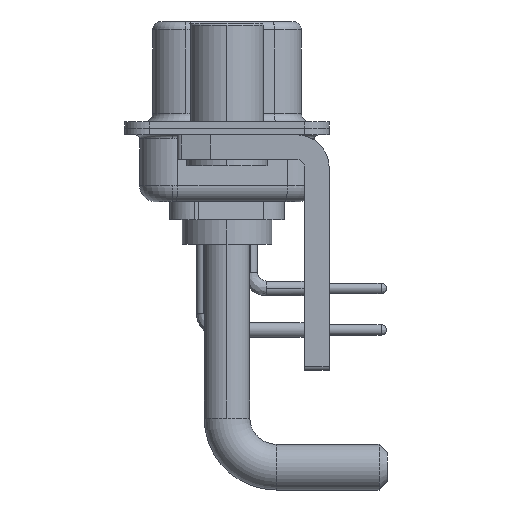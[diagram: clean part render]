
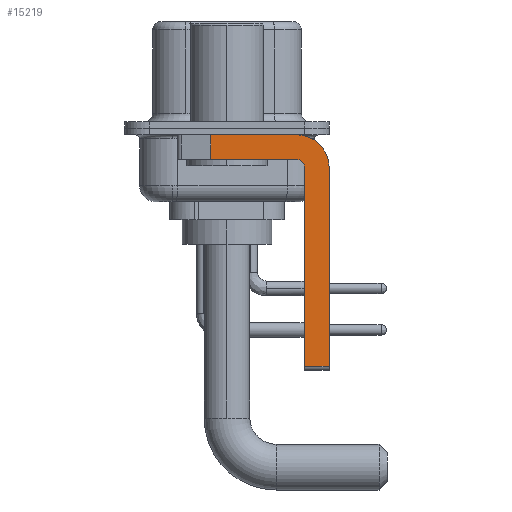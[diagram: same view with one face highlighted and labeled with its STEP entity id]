
A CAD part, left-side view. The second image highlights one B-rep face of the part: STEP entity #15219.
In plain terms, the highlighted planar face has unit normal (-1, 0, 0).
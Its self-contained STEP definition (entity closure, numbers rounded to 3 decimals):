
#39 = VERTEX_POINT ( 'NONE', #13458 ) ;
#466 = VERTEX_POINT ( 'NONE', #19669 ) ;
#591 = EDGE_CURVE ( 'NONE', #25137, #39, #25236, .T. ) ;
#1437 = DIRECTION ( 'NONE',  ( 0., 0., -1. ) ) ;
#1452 = EDGE_CURVE ( 'NONE', #3935, #466, #29299, .T. ) ;
#1576 = VERTEX_POINT ( 'NONE', #20144 ) ;
#1578 = PLANE ( 'NONE',  #26628 ) ;
#1872 = ORIENTED_EDGE ( 'NONE', *, *, #3422, .F. ) ;
#2029 = VERTEX_POINT ( 'NONE', #25623 ) ;
#2745 = VERTEX_POINT ( 'NONE', #3814 ) ;
#3008 = DIRECTION ( 'NONE',  ( 0., 0., -1. ) ) ;
#3422 = EDGE_CURVE ( 'NONE', #1576, #10425, #16753, .T. ) ;
#3678 = DIRECTION ( 'NONE',  ( 1., 0., 0. ) ) ;
#3814 = CARTESIAN_POINT ( 'NONE',  ( -2.9, -6.25, -14.55 ) ) ;
#3935 = VERTEX_POINT ( 'NONE', #21725 ) ;
#3974 = DIRECTION ( 'NONE',  ( 0., 1., 0. ) ) ;
#4480 = CIRCLE ( 'NONE', #8739, 2. ) ;
#4920 = ORIENTED_EDGE ( 'NONE', *, *, #23423, .F. ) ;
#5071 = AXIS2_PLACEMENT_3D ( 'NONE', #21309, #20336, #18812 ) ;
#6153 = EDGE_CURVE ( 'NONE', #10425, #2029, #4480, .T. ) ;
#6484 = CIRCLE ( 'NONE', #5071, 0.5 ) ;
#6546 = EDGE_CURVE ( 'NONE', #1576, #466, #14475, .T. ) ;
#6568 = ORIENTED_EDGE ( 'NONE', *, *, #1452, .F. ) ;
#7498 = ORIENTED_EDGE ( 'NONE', *, *, #591, .F. ) ;
#8739 = AXIS2_PLACEMENT_3D ( 'NONE', #9708, #23617, #3008 ) ;
#8880 = VECTOR ( 'NONE', #9494, 1000. ) ;
#8999 = VECTOR ( 'NONE', #3974, 1000. ) ;
#9494 = DIRECTION ( 'NONE',  ( 0., -1., 0. ) ) ;
#9590 = DIRECTION ( 'NONE',  ( 0., 0., -1. ) ) ;
#9708 = CARTESIAN_POINT ( 'NONE',  ( -2.9, -4.25, -2.4 ) ) ;
#10425 = VERTEX_POINT ( 'NONE', #23174 ) ;
#10518 = ORIENTED_EDGE ( 'NONE', *, *, #24227, .T. ) ;
#11633 = LINE ( 'NONE', #28333, #24427 ) ;
#11795 = CARTESIAN_POINT ( 'NONE',  ( -2.9, 0.978, -1.9 ) ) ;
#13458 = CARTESIAN_POINT ( 'NONE',  ( -2.9, -4.75, -2.4 ) ) ;
#14475 = LINE ( 'NONE', #11795, #28120 ) ;
#14942 = ORIENTED_EDGE ( 'NONE', *, *, #29248, .F. ) ;
#15219 = ADVANCED_FACE ( 'NONE', ( #26167 ), #1578, .F. ) ;
#16158 = CARTESIAN_POINT ( 'NONE',  ( -2.9, -4.25, -14.55 ) ) ;
#16207 = ORIENTED_EDGE ( 'NONE', *, *, #6153, .F. ) ;
#16385 = CARTESIAN_POINT ( 'NONE',  ( -2.9, -4.75, -14.8 ) ) ;
#16618 = CARTESIAN_POINT ( 'NONE',  ( -2.9, 3., -0.4 ) ) ;
#16753 = LINE ( 'NONE', #16618, #24678 ) ;
#17093 = DIRECTION ( 'NONE',  ( 0., 0., -1. ) ) ;
#17559 = EDGE_LOOP ( 'NONE', ( #1872, #19101, #6568, #14942, #7498, #10518, #4920, #16207 ) ) ;
#18812 = DIRECTION ( 'NONE',  ( 0., 0., 1. ) ) ;
#19101 = ORIENTED_EDGE ( 'NONE', *, *, #6546, .T. ) ;
#19669 = CARTESIAN_POINT ( 'NONE',  ( -2.9, 0.978, -1.9 ) ) ;
#19850 = VECTOR ( 'NONE', #24816, 1000. ) ;
#20144 = CARTESIAN_POINT ( 'NONE',  ( -2.9, 0.978, -0.4 ) ) ;
#20336 = DIRECTION ( 'NONE',  ( -1., 0., 0. ) ) ;
#21309 = CARTESIAN_POINT ( 'NONE',  ( -2.9, -4.25, -2.4 ) ) ;
#21350 = DIRECTION ( 'NONE',  ( 0., -1., 0. ) ) ;
#21725 = CARTESIAN_POINT ( 'NONE',  ( -2.9, -4.25, -1.9 ) ) ;
#23117 = LINE ( 'NONE', #16158, #8880 ) ;
#23174 = CARTESIAN_POINT ( 'NONE',  ( -2.9, -4.25, -0.4 ) ) ;
#23423 = EDGE_CURVE ( 'NONE', #2029, #2745, #11633, .T. ) ;
#23617 = DIRECTION ( 'NONE',  ( 1., 0., 0. ) ) ;
#24227 = EDGE_CURVE ( 'NONE', #25137, #2745, #23117, .T. ) ;
#24427 = VECTOR ( 'NONE', #17093, 1000. ) ;
#24475 = CARTESIAN_POINT ( 'NONE',  ( -2.9, -4.75, -14.55 ) ) ;
#24678 = VECTOR ( 'NONE', #21350, 1000. ) ;
#24816 = DIRECTION ( 'NONE',  ( 0., 0., 1. ) ) ;
#25137 = VERTEX_POINT ( 'NONE', #24475 ) ;
#25236 = LINE ( 'NONE', #16385, #19850 ) ;
#25623 = CARTESIAN_POINT ( 'NONE',  ( -2.9, -6.25, -2.4 ) ) ;
#26167 = FACE_OUTER_BOUND ( 'NONE', #17559, .T. ) ;
#26615 = CARTESIAN_POINT ( 'NONE',  ( -2.9, -4.25, -1.9 ) ) ;
#26628 = AXIS2_PLACEMENT_3D ( 'NONE', #28410, #3678, #1437 ) ;
#28120 = VECTOR ( 'NONE', #9590, 1000. ) ;
#28333 = CARTESIAN_POINT ( 'NONE',  ( -2.9, -6.25, -2.4 ) ) ;
#28410 = CARTESIAN_POINT ( 'NONE',  ( -2.9, -4.25, -2.4 ) ) ;
#29248 = EDGE_CURVE ( 'NONE', #39, #3935, #6484, .T. ) ;
#29299 = LINE ( 'NONE', #26615, #8999 ) ;
